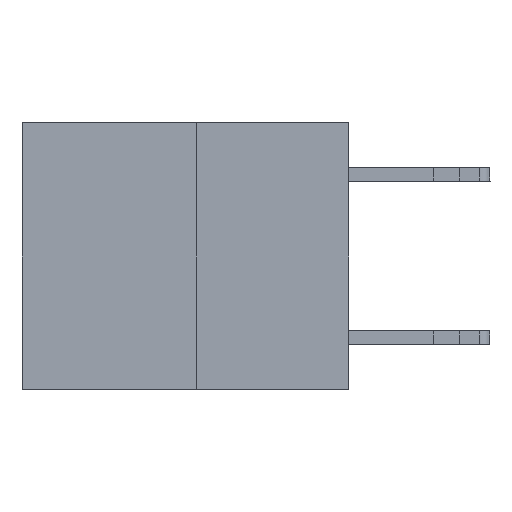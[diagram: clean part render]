
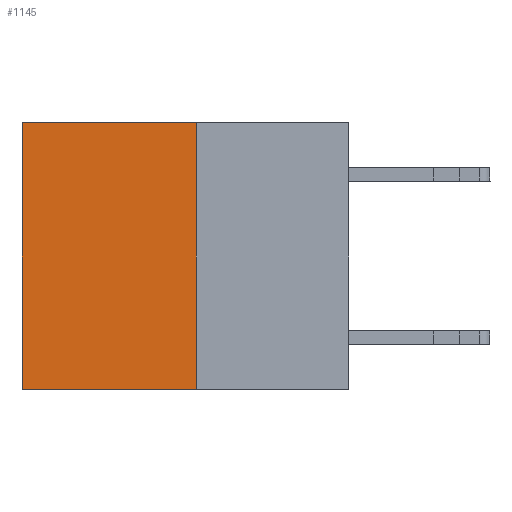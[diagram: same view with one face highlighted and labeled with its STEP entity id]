
A CAD part, left-side view. The second image highlights one B-rep face of the part: STEP entity #1145.
In plain terms, the highlighted planar face has unit normal (-1, 0, 0).
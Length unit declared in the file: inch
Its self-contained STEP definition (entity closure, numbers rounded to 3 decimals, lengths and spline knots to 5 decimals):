
#154 = VECTOR ( 'NONE', #19827, 39.37008 ) ;
#1145 = ADVANCED_FACE ( 'NONE', ( #14195 ), #12845, .F. ) ;
#1780 = CARTESIAN_POINT ( 'NONE',  ( 0.3165, 0.28, -0.49 ) ) ;
#3551 = LINE ( 'NONE', #17828, #154 ) ;
#3732 = DIRECTION ( 'NONE',  ( 0., 1., 0. ) ) ;
#5845 = ORIENTED_EDGE ( 'NONE', *, *, #14678, .T. ) ;
#6097 = VERTEX_POINT ( 'NONE', #12249 ) ;
#8227 = VERTEX_POINT ( 'NONE', #10742 ) ;
#8546 = DIRECTION ( 'NONE',  ( 0., 0., -1. ) ) ;
#8820 = LINE ( 'NONE', #18100, #16497 ) ;
#9246 = ORIENTED_EDGE ( 'NONE', *, *, #24866, .T. ) ;
#10742 = CARTESIAN_POINT ( 'NONE',  ( 0.3165, 0.28, -0.49 ) ) ;
#11079 = VECTOR ( 'NONE', #3732, 39.37008 ) ;
#12249 = CARTESIAN_POINT ( 'NONE',  ( 0.3165, 0.6, 0. ) ) ;
#12845 = PLANE ( 'NONE',  #19966 ) ;
#14195 = FACE_OUTER_BOUND ( 'NONE', #21629, .T. ) ;
#14340 = CARTESIAN_POINT ( 'NONE',  ( 0.3165, 0.28, 0. ) ) ;
#14577 = DIRECTION ( 'NONE',  ( 0., 1., 0. ) ) ;
#14678 = EDGE_CURVE ( 'NONE', #6097, #24235, #8820, .T. ) ;
#14912 = DIRECTION ( 'NONE',  ( 1., 0., 0. ) ) ;
#15219 = VECTOR ( 'NONE', #14577, 39.37008 ) ;
#15237 = ORIENTED_EDGE ( 'NONE', *, *, #18025, .F. ) ;
#16497 = VECTOR ( 'NONE', #8546, 39.37008 ) ;
#17369 = LINE ( 'NONE', #22167, #15219 ) ;
#17607 = LINE ( 'NONE', #1780, #11079 ) ;
#17828 = CARTESIAN_POINT ( 'NONE',  ( 0.3165, 0.28, -0.49 ) ) ;
#18025 = EDGE_CURVE ( 'NONE', #8227, #24235, #17607, .T. ) ;
#18100 = CARTESIAN_POINT ( 'NONE',  ( 0.3165, 0.6, -0.49 ) ) ;
#18865 = DIRECTION ( 'NONE',  ( 0., 0., -1. ) ) ;
#19827 = DIRECTION ( 'NONE',  ( 0., 0., -1. ) ) ;
#19966 = AXIS2_PLACEMENT_3D ( 'NONE', #24709, #14912, #18865 ) ;
#21629 = EDGE_LOOP ( 'NONE', ( #5845, #15237, #25264, #9246 ) ) ;
#22167 = CARTESIAN_POINT ( 'NONE',  ( 0.3165, 0.28, 0. ) ) ;
#23829 = VERTEX_POINT ( 'NONE', #14340 ) ;
#24235 = VERTEX_POINT ( 'NONE', #25354 ) ;
#24709 = CARTESIAN_POINT ( 'NONE',  ( 0.3165, 0.28, -0.49 ) ) ;
#24798 = EDGE_CURVE ( 'NONE', #23829, #8227, #3551, .T. ) ;
#24866 = EDGE_CURVE ( 'NONE', #23829, #6097, #17369, .T. ) ;
#25264 = ORIENTED_EDGE ( 'NONE', *, *, #24798, .F. ) ;
#25354 = CARTESIAN_POINT ( 'NONE',  ( 0.3165, 0.6, -0.49 ) ) ;
